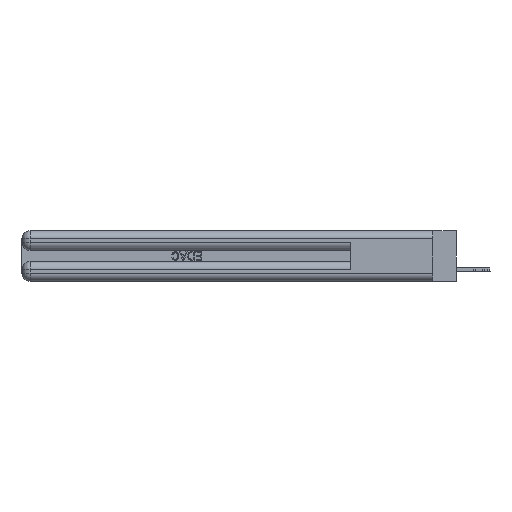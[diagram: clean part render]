
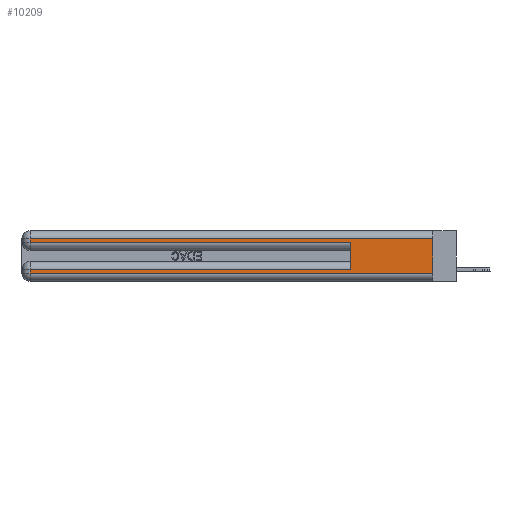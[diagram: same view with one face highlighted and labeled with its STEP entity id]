
A CAD part, left-side view. The second image highlights one B-rep face of the part: STEP entity #10209.
In plain terms, the highlighted planar face has unit normal (-1, 0, 0).
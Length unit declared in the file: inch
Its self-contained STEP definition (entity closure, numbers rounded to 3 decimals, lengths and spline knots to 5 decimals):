
#629 = VECTOR ( 'NONE', #22826, 39.37008 ) ;
#707 = ORIENTED_EDGE ( 'NONE', *, *, #3976, .F. ) ;
#1064 = VECTOR ( 'NONE', #31707, 39.37008 ) ;
#1267 = LINE ( 'NONE', #17000, #49329 ) ;
#2266 = EDGE_CURVE ( 'NONE', #6768, #12939, #9958, .T. ) ;
#2626 = VERTEX_POINT ( 'NONE', #5836 ) ;
#3644 = VECTOR ( 'NONE', #31883, 39.37008 ) ;
#3976 = EDGE_CURVE ( 'NONE', #41237, #22334, #28329, .T. ) ;
#4051 = EDGE_CURVE ( 'NONE', #12939, #22334, #32071, .T. ) ;
#4948 = EDGE_CURVE ( 'NONE', #2626, #18247, #28835, .T. ) ;
#5836 = CARTESIAN_POINT ( 'NONE',  ( 0., 2.94, 0.085 ) ) ;
#6577 = DIRECTION ( 'NONE',  ( 0., 0., -1. ) ) ;
#6768 = VERTEX_POINT ( 'NONE', #17671 ) ;
#7855 = CARTESIAN_POINT ( 'NONE',  ( 0., 0.6, 0.085 ) ) ;
#7947 = CARTESIAN_POINT ( 'NONE',  ( 0., 2.94, 0.06 ) ) ;
#8679 = EDGE_LOOP ( 'NONE', ( #26414, #25152, #35282, #50808, #707, #17901, #42736, #13079 ) ) ;
#9220 = AXIS2_PLACEMENT_3D ( 'NONE', #36704, #46421, #26127 ) ;
#9958 = LINE ( 'NONE', #14472, #19222 ) ;
#10209 = ADVANCED_FACE ( 'NONE', ( #22561 ), #29188, .F. ) ;
#10924 = DIRECTION ( 'NONE',  ( 0., -1., 0. ) ) ;
#11590 = CARTESIAN_POINT ( 'NONE',  ( 0., 2.94, 0.37 ) ) ;
#12862 = DIRECTION ( 'NONE',  ( 0., 0., -1. ) ) ;
#12939 = VERTEX_POINT ( 'NONE', #49833 ) ;
#13079 = ORIENTED_EDGE ( 'NONE', *, *, #44927, .T. ) ;
#14107 = EDGE_CURVE ( 'NONE', #41237, #2626, #50800, .T. ) ;
#14147 = CARTESIAN_POINT ( 'NONE',  ( 0., 0., 0.085 ) ) ;
#14472 = CARTESIAN_POINT ( 'NONE',  ( 0., 2.94, 0.37 ) ) ;
#14948 = VECTOR ( 'NONE', #12862, 39.37008 ) ;
#17000 = CARTESIAN_POINT ( 'NONE',  ( 0., 0., 0.31 ) ) ;
#17671 = CARTESIAN_POINT ( 'NONE',  ( 0., 2.94, 0.31 ) ) ;
#17901 = ORIENTED_EDGE ( 'NONE', *, *, #14107, .T. ) ;
#18247 = VERTEX_POINT ( 'NONE', #7947 ) ;
#19222 = VECTOR ( 'NONE', #6577, 39.37008 ) ;
#19338 = VECTOR ( 'NONE', #49819, 39.37008 ) ;
#21589 = VECTOR ( 'NONE', #10924, 39.37008 ) ;
#22011 = LINE ( 'NONE', #47544, #1064 ) ;
#22334 = VERTEX_POINT ( 'NONE', #28982 ) ;
#22561 = FACE_OUTER_BOUND ( 'NONE', #8679, .T. ) ;
#22607 = CARTESIAN_POINT ( 'NONE',  ( 0., 0., 0.31 ) ) ;
#22826 = DIRECTION ( 'NONE',  ( 0., 0., 1. ) ) ;
#23054 = EDGE_CURVE ( 'NONE', #25170, #38859, #40266, .T. ) ;
#25152 = ORIENTED_EDGE ( 'NONE', *, *, #49499, .T. ) ;
#25170 = VERTEX_POINT ( 'NONE', #22607 ) ;
#25407 = DIRECTION ( 'NONE',  ( 0., 1., 0. ) ) ;
#26127 = DIRECTION ( 'NONE',  ( 0., 0., -1. ) ) ;
#26414 = ORIENTED_EDGE ( 'NONE', *, *, #23054, .F. ) ;
#28329 = LINE ( 'NONE', #46236, #629 ) ;
#28835 = LINE ( 'NONE', #11590, #3644 ) ;
#28982 = CARTESIAN_POINT ( 'NONE',  ( 0., 0.6, 0.285 ) ) ;
#29188 = PLANE ( 'NONE',  #9220 ) ;
#31707 = DIRECTION ( 'NONE',  ( 0., -1., 0. ) ) ;
#31883 = DIRECTION ( 'NONE',  ( 0., 0., -1. ) ) ;
#32071 = LINE ( 'NONE', #34551, #21589 ) ;
#34551 = CARTESIAN_POINT ( 'NONE',  ( 0., 0., 0.285 ) ) ;
#35282 = ORIENTED_EDGE ( 'NONE', *, *, #2266, .T. ) ;
#36704 = CARTESIAN_POINT ( 'NONE',  ( 0., 0., 0.37 ) ) ;
#38859 = VERTEX_POINT ( 'NONE', #50587 ) ;
#40266 = LINE ( 'NONE', #48626, #14948 ) ;
#41237 = VERTEX_POINT ( 'NONE', #7855 ) ;
#42736 = ORIENTED_EDGE ( 'NONE', *, *, #4948, .T. ) ;
#44927 = EDGE_CURVE ( 'NONE', #18247, #38859, #22011, .T. ) ;
#46236 = CARTESIAN_POINT ( 'NONE',  ( 0., 0.6, 0.145 ) ) ;
#46421 = DIRECTION ( 'NONE',  ( 1., 0., 0. ) ) ;
#47544 = CARTESIAN_POINT ( 'NONE',  ( 0., 0., 0.06 ) ) ;
#48626 = CARTESIAN_POINT ( 'NONE',  ( 0., 0., 0.37 ) ) ;
#49329 = VECTOR ( 'NONE', #25407, 39.37008 ) ;
#49499 = EDGE_CURVE ( 'NONE', #25170, #6768, #1267, .T. ) ;
#49819 = DIRECTION ( 'NONE',  ( 0., 1., 0. ) ) ;
#49833 = CARTESIAN_POINT ( 'NONE',  ( 0., 2.94, 0.285 ) ) ;
#50587 = CARTESIAN_POINT ( 'NONE',  ( 0., 0., 0.06 ) ) ;
#50800 = LINE ( 'NONE', #14147, #19338 ) ;
#50808 = ORIENTED_EDGE ( 'NONE', *, *, #4051, .T. ) ;
